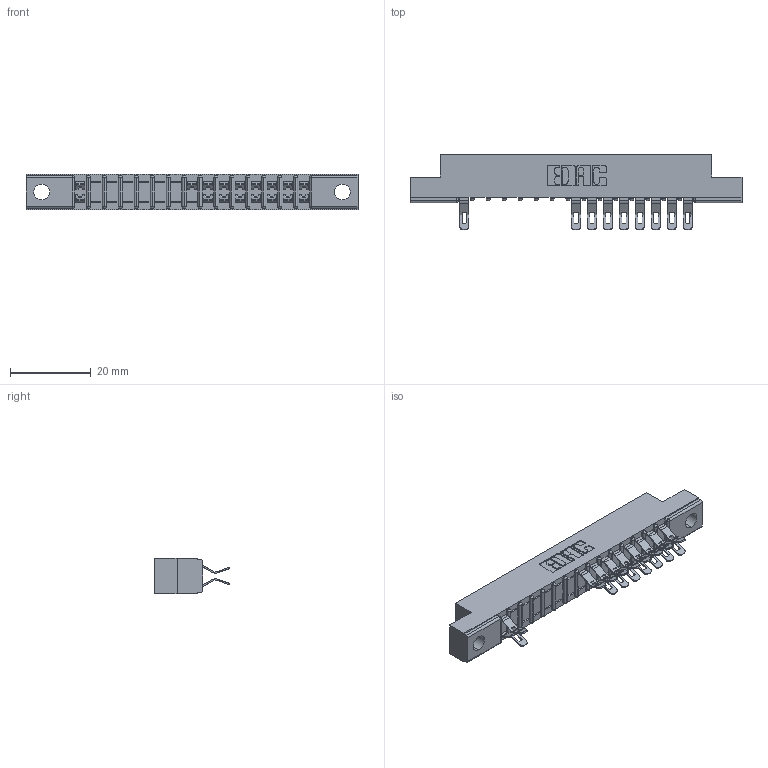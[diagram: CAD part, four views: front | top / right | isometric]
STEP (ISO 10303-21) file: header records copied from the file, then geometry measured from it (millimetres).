
FILE_DESCRIPTION (( 'STEP AP203' ), '1' );
FILE_NAME ('307-030-555-202.STEP', '2018-08-04T19:43:24', ( '' ), ( '' ), 'SwSTEP 2.0', 'SolidWorks 2016', '' );
FILE_SCHEMA (( 'CONFIG_CONTROL_DESIGN' ));
Length unit declared in the file: inch
Products named in the file (3): 307 Part_.128 Dia Mounting Holes; 307-290-001_555; 307-030-555-202
Assembly tree (18 placements, depth 2):
  307-030-555-202
    307 Part_.128 Dia Mounting Holes
    307-290-001_555  x17
Bounding box: 82.45 x 18.75 x 8.71 mm (x, y, z)
Volume: 5188.3 mm3; surface area: 7931.3 mm2
Topology: 18 solids, 18 shells, 1301 faces, 3816 edges, 2476 vertices
Faces by surface type: plane 726, cylinder 543, sphere 32
Entity records: 16791 total; most frequent: CARTESIAN_POINT 2814, ORIENTED_EDGE 2800, DIRECTION 2762, EDGE_CURVE 1400, LINE 1050, VECTOR 1050, VERTEX_POINT 908, AXIS2_PLACEMENT_3D 856
